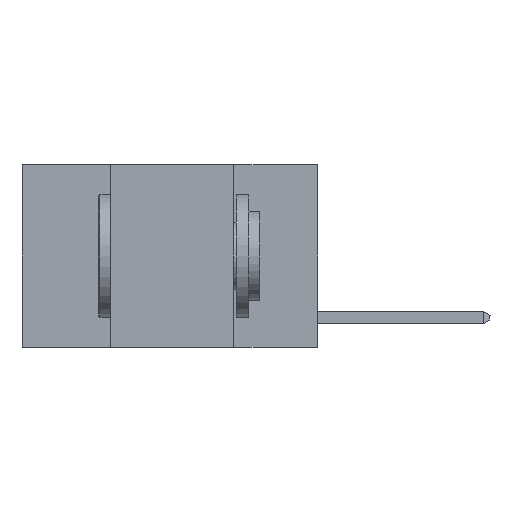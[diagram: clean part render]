
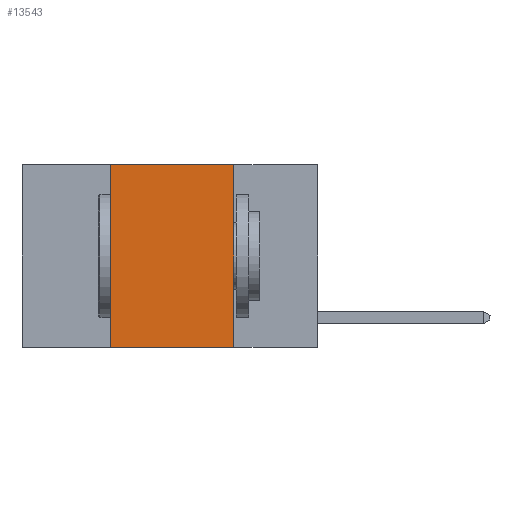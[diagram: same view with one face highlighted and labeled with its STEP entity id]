
A CAD part, left-side view. The second image highlights one B-rep face of the part: STEP entity #13543.
In plain terms, the highlighted planar face has unit normal (-1, 0, 0).
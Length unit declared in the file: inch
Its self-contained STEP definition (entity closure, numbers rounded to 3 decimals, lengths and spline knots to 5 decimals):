
#96 = VERTEX_POINT ( 'NONE', #6205 ) ;
#958 = LINE ( 'NONE', #10303, #23087 ) ;
#1220 = ORIENTED_EDGE ( 'NONE', *, *, #17546, .F. ) ;
#1310 = CARTESIAN_POINT ( 'NONE',  ( 0., 0.17, 0. ) ) ;
#3217 = ORIENTED_EDGE ( 'NONE', *, *, #21588, .F. ) ;
#3601 = VERTEX_POINT ( 'NONE', #24444 ) ;
#4432 = LINE ( 'NONE', #23099, #11252 ) ;
#6205 = CARTESIAN_POINT ( 'NONE',  ( 0., 0.42, -0.37 ) ) ;
#7038 = DIRECTION ( 'NONE',  ( 0., -1., 0. ) ) ;
#7549 = EDGE_CURVE ( 'NONE', #96, #3601, #958, .T. ) ;
#8660 = LINE ( 'NONE', #27151, #9011 ) ;
#9011 = VECTOR ( 'NONE', #22283, 39.37008 ) ;
#10170 = VECTOR ( 'NONE', #23322, 39.37008 ) ;
#10303 = CARTESIAN_POINT ( 'NONE',  ( 0., 0.6, -0.37 ) ) ;
#11252 = VECTOR ( 'NONE', #7038, 39.37008 ) ;
#12165 = ORIENTED_EDGE ( 'NONE', *, *, #23855, .F. ) ;
#13543 = ADVANCED_FACE ( 'NONE', ( #21905 ), #17484, .F. ) ;
#13690 = CARTESIAN_POINT ( 'NONE',  ( 0., 0.17, 0. ) ) ;
#14726 = CARTESIAN_POINT ( 'NONE',  ( 0., 0.6, 0. ) ) ;
#14856 = ORIENTED_EDGE ( 'NONE', *, *, #7549, .T. ) ;
#16051 = CARTESIAN_POINT ( 'NONE',  ( 0., 0.42, 0. ) ) ;
#17484 = PLANE ( 'NONE',  #28406 ) ;
#17546 = EDGE_CURVE ( 'NONE', #96, #22873, #8660, .T. ) ;
#20573 = LINE ( 'NONE', #13690, #10170 ) ;
#21588 = EDGE_CURVE ( 'NONE', #28289, #3601, #20573, .T. ) ;
#21616 = EDGE_LOOP ( 'NONE', ( #3217, #12165, #1220, #14856 ) ) ;
#21905 = FACE_OUTER_BOUND ( 'NONE', #21616, .T. ) ;
#22283 = DIRECTION ( 'NONE',  ( 0., 0., 1. ) ) ;
#22873 = VERTEX_POINT ( 'NONE', #16051 ) ;
#23087 = VECTOR ( 'NONE', #29102, 39.37008 ) ;
#23099 = CARTESIAN_POINT ( 'NONE',  ( 0., 0.6, 0. ) ) ;
#23322 = DIRECTION ( 'NONE',  ( 0., 0., -1. ) ) ;
#23855 = EDGE_CURVE ( 'NONE', #22873, #28289, #4432, .T. ) ;
#24032 = DIRECTION ( 'NONE',  ( 1., 0., 0. ) ) ;
#24444 = CARTESIAN_POINT ( 'NONE',  ( 0., 0.17, -0.37 ) ) ;
#24477 = DIRECTION ( 'NONE',  ( 0., 0., -1. ) ) ;
#27151 = CARTESIAN_POINT ( 'NONE',  ( 0., 0.42, 0. ) ) ;
#28289 = VERTEX_POINT ( 'NONE', #1310 ) ;
#28406 = AXIS2_PLACEMENT_3D ( 'NONE', #14726, #24032, #24477 ) ;
#29102 = DIRECTION ( 'NONE',  ( 0., -1., 0. ) ) ;
